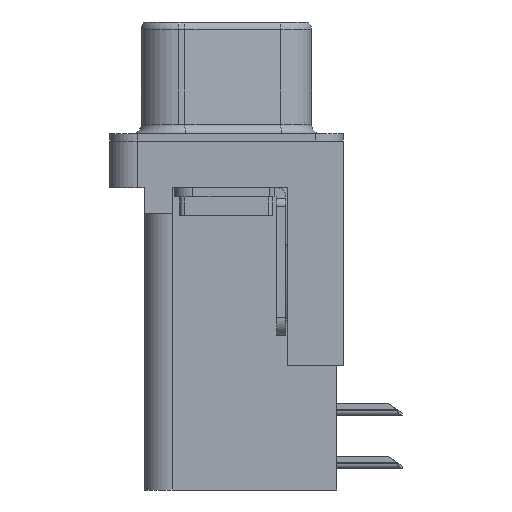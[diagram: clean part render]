
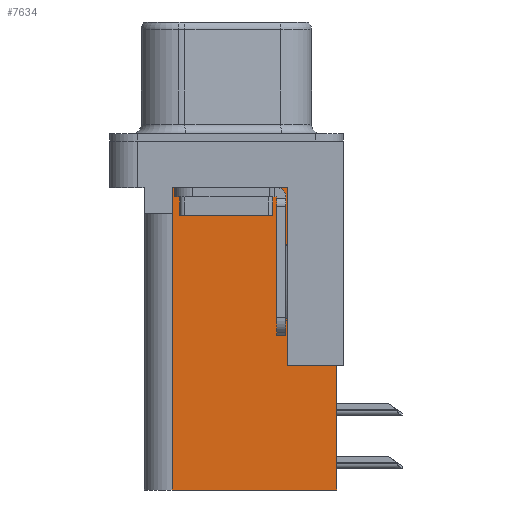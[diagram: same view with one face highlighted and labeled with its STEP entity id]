
A CAD part, left-side view. The second image highlights one B-rep face of the part: STEP entity #7634.
In plain terms, the highlighted planar face has unit normal (-1, 0, 0).
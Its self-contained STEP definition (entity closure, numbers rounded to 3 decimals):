
#1447 = CARTESIAN_POINT ( 'NONE',  ( 3.79, -3.295, -18.76 ) ) ;
#1950 = LINE ( 'NONE', #14827, #24232 ) ;
#3051 = CARTESIAN_POINT ( 'NONE',  ( 3.79, 2.925, -3.9 ) ) ;
#3173 = LINE ( 'NONE', #13177, #14317 ) ;
#3320 = EDGE_CURVE ( 'NONE', #11576, #7203, #13558, .T. ) ;
#3662 = AXIS2_PLACEMENT_3D ( 'NONE', #5194, #7363, #22936 ) ;
#4452 = ORIENTED_EDGE ( 'NONE', *, *, #24591, .T. ) ;
#4454 = CARTESIAN_POINT ( 'NONE',  ( 3.79, 2.925, -18.76 ) ) ;
#5194 = CARTESIAN_POINT ( 'NONE',  ( 3.79, -3.295, -18.76 ) ) ;
#5200 = VECTOR ( 'NONE', #14538, 1000. ) ;
#6201 = CARTESIAN_POINT ( 'NONE',  ( 3.79, -6.295, -12.05 ) ) ;
#6532 = CARTESIAN_POINT ( 'NONE',  ( 3.79, -5.925, -18.76 ) ) ;
#6657 = VECTOR ( 'NONE', #12381, 1000. ) ;
#7203 = VERTEX_POINT ( 'NONE', #3051 ) ;
#7363 = DIRECTION ( 'NONE',  ( 1., 0., 0. ) ) ;
#7465 = VECTOR ( 'NONE', #23716, 1000. ) ;
#7634 = ADVANCED_FACE ( 'NONE', ( #15474 ), #18461, .F. ) ;
#7750 = CARTESIAN_POINT ( 'NONE',  ( 3.79, 2.895, -2.5 ) ) ;
#7974 = VECTOR ( 'NONE', #26281, 1000. ) ;
#8108 = EDGE_LOOP ( 'NONE', ( #24497, #20096, #26052, #8484, #25350, #8912, #12696, #4452 ) ) ;
#8484 = ORIENTED_EDGE ( 'NONE', *, *, #3320, .F. ) ;
#8513 = CARTESIAN_POINT ( 'NONE',  ( 3.79, -5.925, -12.05 ) ) ;
#8770 = CARTESIAN_POINT ( 'NONE',  ( 3.79, -3.295, -2.5 ) ) ;
#8912 = ORIENTED_EDGE ( 'NONE', *, *, #26299, .F. ) ;
#9226 = EDGE_CURVE ( 'NONE', #22749, #13837, #1950, .T. ) ;
#10495 = CARTESIAN_POINT ( 'NONE',  ( 3.79, -5.925, -2. ) ) ;
#11576 = VERTEX_POINT ( 'NONE', #4454 ) ;
#11676 = CARTESIAN_POINT ( 'NONE',  ( 3.79, 2.925, -18.76 ) ) ;
#12381 = DIRECTION ( 'NONE',  ( 0., 1., 0. ) ) ;
#12542 = DIRECTION ( 'NONE',  ( 0., 0., -1. ) ) ;
#12696 = ORIENTED_EDGE ( 'NONE', *, *, #14340, .T. ) ;
#12773 = EDGE_CURVE ( 'NONE', #18797, #22749, #24725, .T. ) ;
#13177 = CARTESIAN_POINT ( 'NONE',  ( 3.79, -3.295, -18.76 ) ) ;
#13420 = LINE ( 'NONE', #1447, #7465 ) ;
#13445 = DIRECTION ( 'NONE',  ( 0., 0., 1. ) ) ;
#13558 = LINE ( 'NONE', #11676, #19464 ) ;
#13837 = VERTEX_POINT ( 'NONE', #15740 ) ;
#13887 = LINE ( 'NONE', #6201, #7974 ) ;
#14023 = VECTOR ( 'NONE', #23852, 1000. ) ;
#14317 = VECTOR ( 'NONE', #26561, 1000. ) ;
#14340 = EDGE_CURVE ( 'NONE', #15853, #20624, #13887, .T. ) ;
#14538 = DIRECTION ( 'NONE',  ( 0., 1., 0. ) ) ;
#14827 = CARTESIAN_POINT ( 'NONE',  ( 3.79, 2.895, -3.9 ) ) ;
#14830 = CARTESIAN_POINT ( 'NONE',  ( 3.79, -3.295, -12.05 ) ) ;
#15066 = EDGE_CURVE ( 'NONE', #13837, #7203, #16295, .T. ) ;
#15474 = FACE_OUTER_BOUND ( 'NONE', #8108, .T. ) ;
#15740 = CARTESIAN_POINT ( 'NONE',  ( 3.79, 2.895, -3.9 ) ) ;
#15853 = VERTEX_POINT ( 'NONE', #8513 ) ;
#16295 = LINE ( 'NONE', #27870, #5200 ) ;
#18461 = PLANE ( 'NONE',  #3662 ) ;
#18517 = LINE ( 'NONE', #10495, #14023 ) ;
#18769 = EDGE_CURVE ( 'NONE', #23544, #11576, #3173, .T. ) ;
#18797 = VERTEX_POINT ( 'NONE', #8770 ) ;
#18999 = CARTESIAN_POINT ( 'NONE',  ( 3.79, -3.295, -2.5 ) ) ;
#19464 = VECTOR ( 'NONE', #13445, 1000. ) ;
#20096 = ORIENTED_EDGE ( 'NONE', *, *, #9226, .T. ) ;
#20624 = VERTEX_POINT ( 'NONE', #14830 ) ;
#22749 = VERTEX_POINT ( 'NONE', #7750 ) ;
#22936 = DIRECTION ( 'NONE',  ( 0., 1., 0. ) ) ;
#23544 = VERTEX_POINT ( 'NONE', #6532 ) ;
#23716 = DIRECTION ( 'NONE',  ( 0., 0., 1. ) ) ;
#23852 = DIRECTION ( 'NONE',  ( 0., 0., -1. ) ) ;
#24232 = VECTOR ( 'NONE', #12542, 1000. ) ;
#24497 = ORIENTED_EDGE ( 'NONE', *, *, #12773, .T. ) ;
#24591 = EDGE_CURVE ( 'NONE', #20624, #18797, #13420, .T. ) ;
#24725 = LINE ( 'NONE', #18999, #6657 ) ;
#25350 = ORIENTED_EDGE ( 'NONE', *, *, #18769, .F. ) ;
#26052 = ORIENTED_EDGE ( 'NONE', *, *, #15066, .T. ) ;
#26281 = DIRECTION ( 'NONE',  ( 0., 1., 0. ) ) ;
#26299 = EDGE_CURVE ( 'NONE', #15853, #23544, #18517, .T. ) ;
#26561 = DIRECTION ( 'NONE',  ( 0., 1., 0. ) ) ;
#27870 = CARTESIAN_POINT ( 'NONE',  ( 3.79, 0., -3.9 ) ) ;
